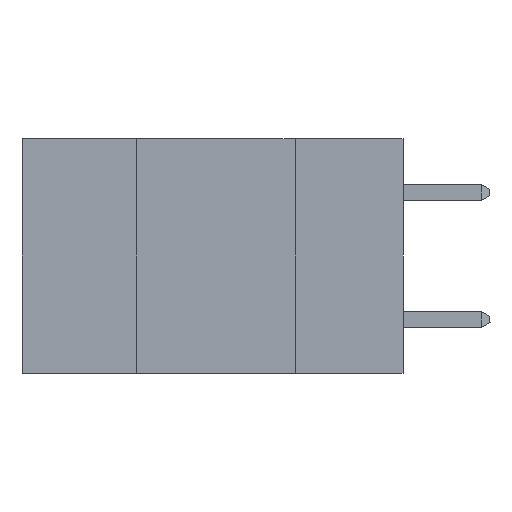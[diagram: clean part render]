
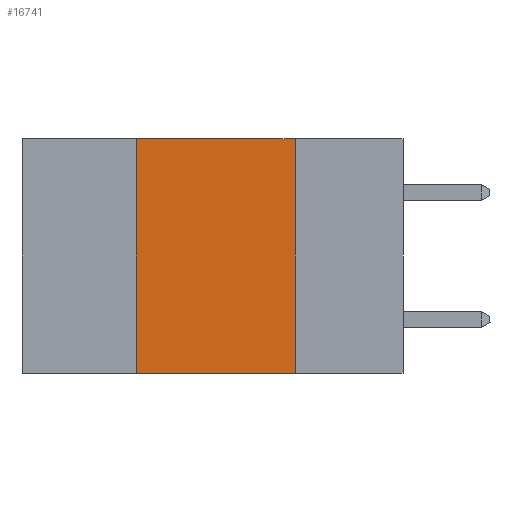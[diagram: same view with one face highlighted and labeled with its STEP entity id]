
A CAD part, left-side view. The second image highlights one B-rep face of the part: STEP entity #16741.
In plain terms, the highlighted planar face has unit normal (-1, 0, 0).
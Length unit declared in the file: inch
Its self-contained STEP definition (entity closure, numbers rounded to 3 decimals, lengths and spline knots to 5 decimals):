
#10 = DIRECTION ( 'NONE',  ( 0., -1., 0. ) ) ;
#809 = CARTESIAN_POINT ( 'NONE',  ( 0., 0.42, 0. ) ) ;
#1679 = EDGE_CURVE ( 'NONE', #10453, #31467, #6894, .T. ) ;
#3886 = VECTOR ( 'NONE', #10, 39.37008 ) ;
#5012 = EDGE_CURVE ( 'NONE', #26867, #16664, #19144, .T. ) ;
#5197 = ORIENTED_EDGE ( 'NONE', *, *, #1679, .F. ) ;
#6423 = DIRECTION ( 'NONE',  ( 0., 0., 1. ) ) ;
#6894 = LINE ( 'NONE', #25217, #29739 ) ;
#6909 = VECTOR ( 'NONE', #6423, 39.37008 ) ;
#8001 = EDGE_CURVE ( 'NONE', #16664, #10453, #16441, .T. ) ;
#8441 = CARTESIAN_POINT ( 'NONE',  ( 0., 0.6, 0. ) ) ;
#10453 = VERTEX_POINT ( 'NONE', #27228 ) ;
#12927 = CARTESIAN_POINT ( 'NONE',  ( 0., 0.17, -0.37 ) ) ;
#13748 = AXIS2_PLACEMENT_3D ( 'NONE', #8441, #31214, #26772 ) ;
#14399 = ORIENTED_EDGE ( 'NONE', *, *, #5012, .F. ) ;
#16441 = LINE ( 'NONE', #16763, #24457 ) ;
#16664 = VERTEX_POINT ( 'NONE', #20512 ) ;
#16741 = ADVANCED_FACE ( 'NONE', ( #31372 ), #31714, .F. ) ;
#16763 = CARTESIAN_POINT ( 'NONE',  ( 0., 0.6, 0. ) ) ;
#17546 = EDGE_CURVE ( 'NONE', #26867, #31467, #30598, .T. ) ;
#19144 = LINE ( 'NONE', #809, #6909 ) ;
#20383 = CARTESIAN_POINT ( 'NONE',  ( 0., 0.6, -0.37 ) ) ;
#20512 = CARTESIAN_POINT ( 'NONE',  ( 0., 0.42, 0. ) ) ;
#22307 = CARTESIAN_POINT ( 'NONE',  ( 0., 0.42, -0.37 ) ) ;
#24233 = DIRECTION ( 'NONE',  ( 0., 0., -1. ) ) ;
#24241 = EDGE_LOOP ( 'NONE', ( #5197, #28982, #14399, #25243 ) ) ;
#24457 = VECTOR ( 'NONE', #27113, 39.37008 ) ;
#25217 = CARTESIAN_POINT ( 'NONE',  ( 0., 0.17, 0. ) ) ;
#25243 = ORIENTED_EDGE ( 'NONE', *, *, #17546, .T. ) ;
#26772 = DIRECTION ( 'NONE',  ( 0., 0., -1. ) ) ;
#26867 = VERTEX_POINT ( 'NONE', #22307 ) ;
#27113 = DIRECTION ( 'NONE',  ( 0., -1., 0. ) ) ;
#27228 = CARTESIAN_POINT ( 'NONE',  ( 0., 0.17, 0. ) ) ;
#28982 = ORIENTED_EDGE ( 'NONE', *, *, #8001, .F. ) ;
#29739 = VECTOR ( 'NONE', #24233, 39.37008 ) ;
#30598 = LINE ( 'NONE', #20383, #3886 ) ;
#31214 = DIRECTION ( 'NONE',  ( 1., 0., 0. ) ) ;
#31372 = FACE_OUTER_BOUND ( 'NONE', #24241, .T. ) ;
#31467 = VERTEX_POINT ( 'NONE', #12927 ) ;
#31714 = PLANE ( 'NONE',  #13748 ) ;
